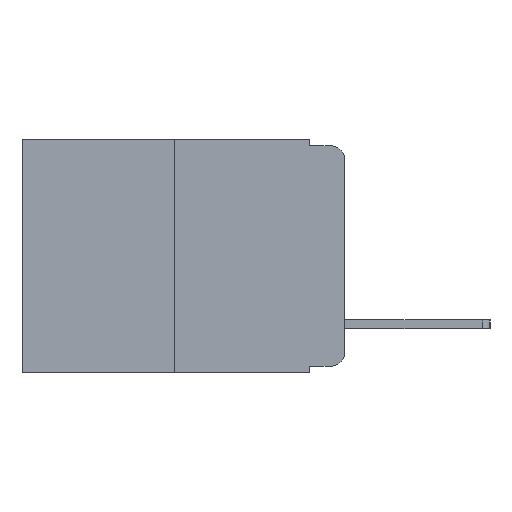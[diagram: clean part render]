
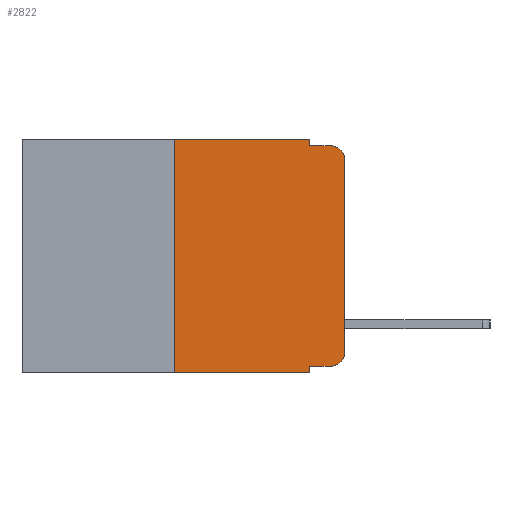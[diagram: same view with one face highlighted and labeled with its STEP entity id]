
A CAD part, left-side view. The second image highlights one B-rep face of the part: STEP entity #2822.
In plain terms, the highlighted planar face has unit normal (-1, 0, 0).
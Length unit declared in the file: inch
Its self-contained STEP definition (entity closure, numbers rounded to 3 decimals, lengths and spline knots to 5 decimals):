
#38 = ORIENTED_EDGE ( 'NONE', *, *, #5863, .F. ) ;
#343 = DIRECTION ( 'NONE',  ( 0., 0., -1. ) ) ;
#407 = ORIENTED_EDGE ( 'NONE', *, *, #5943, .T. ) ;
#591 = VECTOR ( 'NONE', #9529, 39.37008 ) ;
#609 = CARTESIAN_POINT ( 'NONE',  ( 0., 0.473, -0.343 ) ) ;
#986 = CARTESIAN_POINT ( 'NONE',  ( 0., 0.25, 0. ) ) ;
#1160 = VERTEX_POINT ( 'NONE', #3758 ) ;
#1240 = CARTESIAN_POINT ( 'NONE',  ( 0., 0.051, -0.01 ) ) ;
#1256 = VECTOR ( 'NONE', #8555, 39.37008 ) ;
#1271 = CARTESIAN_POINT ( 'NONE',  ( 0., 0., -0.313 ) ) ;
#1352 = EDGE_CURVE ( 'NONE', #5347, #5237, #8110, .T. ) ;
#1367 = PLANE ( 'NONE',  #6410 ) ;
#1548 = EDGE_CURVE ( 'NONE', #6540, #1160, #3922, .T. ) ;
#2297 = LINE ( 'NONE', #609, #6575 ) ;
#2378 = VERTEX_POINT ( 'NONE', #2691 ) ;
#2403 = DIRECTION ( 'NONE',  ( 0., 0., -1. ) ) ;
#2411 = CARTESIAN_POINT ( 'NONE',  ( 0., 0.051, -0.01 ) ) ;
#2672 = DIRECTION ( 'NONE',  ( 0., -1., 0. ) ) ;
#2691 = CARTESIAN_POINT ( 'NONE',  ( 0., 0.051, 0. ) ) ;
#2728 = CARTESIAN_POINT ( 'NONE',  ( 0., 0.02, -0.01 ) ) ;
#2822 = ADVANCED_FACE ( 'NONE', ( #7536 ), #1367, .F. ) ;
#2843 = VERTEX_POINT ( 'NONE', #5223 ) ;
#3229 = EDGE_CURVE ( 'NONE', #2843, #6132, #4977, .T. ) ;
#3758 = CARTESIAN_POINT ( 'NONE',  ( 0., 0.02, -0.333 ) ) ;
#3793 = CIRCLE ( 'NONE', #6426, 0.02 ) ;
#3922 = LINE ( 'NONE', #6004, #1256 ) ;
#3932 = LINE ( 'NONE', #8677, #591 ) ;
#4360 = ORIENTED_EDGE ( 'NONE', *, *, #6781, .F. ) ;
#4402 = EDGE_CURVE ( 'NONE', #5347, #10364, #2297, .T. ) ;
#4658 = CARTESIAN_POINT ( 'NONE',  ( 0., 0.25, -0.343 ) ) ;
#4892 = ORIENTED_EDGE ( 'NONE', *, *, #11716, .F. ) ;
#4975 = CARTESIAN_POINT ( 'NONE',  ( 0., 0.051, -0.333 ) ) ;
#4977 = CIRCLE ( 'NONE', #8844, 0.02 ) ;
#5203 = VECTOR ( 'NONE', #5433, 39.37008 ) ;
#5210 = EDGE_CURVE ( 'NONE', #6540, #10364, #9987, .T. ) ;
#5223 = CARTESIAN_POINT ( 'NONE',  ( 0., 0., -0.03 ) ) ;
#5237 = VERTEX_POINT ( 'NONE', #8865 ) ;
#5305 = DIRECTION ( 'NONE',  ( -1., 0., 0. ) ) ;
#5310 = DIRECTION ( 'NONE',  ( 0., 0., 1. ) ) ;
#5347 = VERTEX_POINT ( 'NONE', #4658 ) ;
#5433 = DIRECTION ( 'NONE',  ( 0., 0., -1. ) ) ;
#5776 = VERTEX_POINT ( 'NONE', #1240 ) ;
#5817 = ORIENTED_EDGE ( 'NONE', *, *, #1352, .F. ) ;
#5863 = EDGE_CURVE ( 'NONE', #5776, #6132, #9197, .T. ) ;
#5943 = EDGE_CURVE ( 'NONE', #1160, #9063, #3793, .T. ) ;
#6004 = CARTESIAN_POINT ( 'NONE',  ( 0., 0.051, -0.333 ) ) ;
#6081 = DIRECTION ( 'NONE',  ( -1., 0., 0. ) ) ;
#6132 = VERTEX_POINT ( 'NONE', #2728 ) ;
#6162 = EDGE_LOOP ( 'NONE', ( #8075, #8209, #38, #4360, #4892, #5817, #10939, #11610, #9666, #407 ) ) ;
#6390 = CARTESIAN_POINT ( 'NONE',  ( 0., 0.051, -0.343 ) ) ;
#6410 = AXIS2_PLACEMENT_3D ( 'NONE', #9422, #7759, #2403 ) ;
#6426 = AXIS2_PLACEMENT_3D ( 'NONE', #10396, #5305, #11263 ) ;
#6540 = VERTEX_POINT ( 'NONE', #4975 ) ;
#6575 = VECTOR ( 'NONE', #2672, 39.37008 ) ;
#6596 = DIRECTION ( 'NONE',  ( 0., 0., 1. ) ) ;
#6781 = EDGE_CURVE ( 'NONE', #2378, #5776, #3932, .T. ) ;
#6790 = LINE ( 'NONE', #7841, #11042 ) ;
#6932 = VECTOR ( 'NONE', #9470, 39.37008 ) ;
#7536 = FACE_OUTER_BOUND ( 'NONE', #6162, .T. ) ;
#7706 = VECTOR ( 'NONE', #11135, 39.37008 ) ;
#7759 = DIRECTION ( 'NONE',  ( 1., 0., 0. ) ) ;
#7841 = CARTESIAN_POINT ( 'NONE',  ( 0., 0., 0. ) ) ;
#7981 = LINE ( 'NONE', #9381, #7706 ) ;
#8075 = ORIENTED_EDGE ( 'NONE', *, *, #11243, .T. ) ;
#8110 = LINE ( 'NONE', #986, #10085 ) ;
#8209 = ORIENTED_EDGE ( 'NONE', *, *, #3229, .T. ) ;
#8555 = DIRECTION ( 'NONE',  ( 0., -1., 0. ) ) ;
#8677 = CARTESIAN_POINT ( 'NONE',  ( 0., 0.051, 0. ) ) ;
#8844 = AXIS2_PLACEMENT_3D ( 'NONE', #11164, #6081, #343 ) ;
#8865 = CARTESIAN_POINT ( 'NONE',  ( 0., 0.25, 0. ) ) ;
#9063 = VERTEX_POINT ( 'NONE', #1271 ) ;
#9197 = LINE ( 'NONE', #2411, #6932 ) ;
#9381 = CARTESIAN_POINT ( 'NONE',  ( 0., 0.473, 0. ) ) ;
#9422 = CARTESIAN_POINT ( 'NONE',  ( 0., 0.473, 0. ) ) ;
#9470 = DIRECTION ( 'NONE',  ( 0., -1., 0. ) ) ;
#9529 = DIRECTION ( 'NONE',  ( 0., 0., -1. ) ) ;
#9666 = ORIENTED_EDGE ( 'NONE', *, *, #1548, .T. ) ;
#9987 = LINE ( 'NONE', #10489, #5203 ) ;
#10085 = VECTOR ( 'NONE', #6596, 39.37008 ) ;
#10364 = VERTEX_POINT ( 'NONE', #6390 ) ;
#10396 = CARTESIAN_POINT ( 'NONE',  ( 0., 0.02, -0.313 ) ) ;
#10489 = CARTESIAN_POINT ( 'NONE',  ( 0., 0.051, 0. ) ) ;
#10939 = ORIENTED_EDGE ( 'NONE', *, *, #4402, .T. ) ;
#11042 = VECTOR ( 'NONE', #5310, 39.37008 ) ;
#11135 = DIRECTION ( 'NONE',  ( 0., -1., 0. ) ) ;
#11164 = CARTESIAN_POINT ( 'NONE',  ( 0., 0.02, -0.03 ) ) ;
#11243 = EDGE_CURVE ( 'NONE', #9063, #2843, #6790, .T. ) ;
#11263 = DIRECTION ( 'NONE',  ( 0., 0., -1. ) ) ;
#11610 = ORIENTED_EDGE ( 'NONE', *, *, #5210, .F. ) ;
#11716 = EDGE_CURVE ( 'NONE', #5237, #2378, #7981, .T. ) ;
